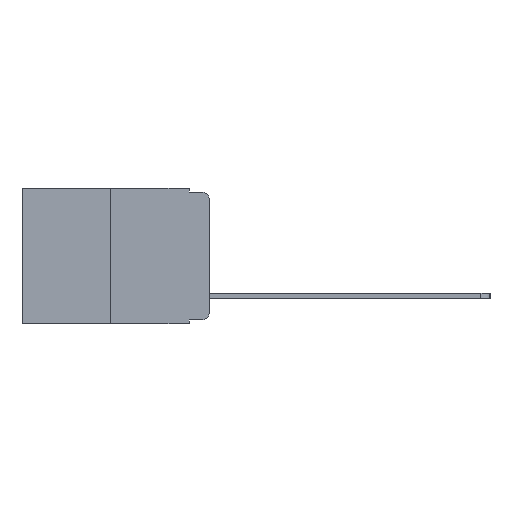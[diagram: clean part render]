
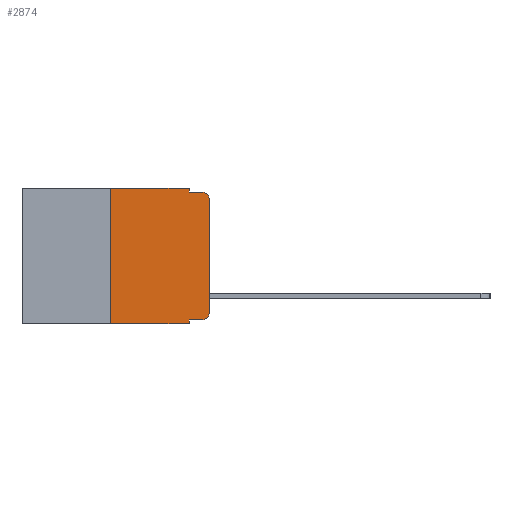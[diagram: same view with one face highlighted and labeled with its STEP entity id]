
A CAD part, left-side view. The second image highlights one B-rep face of the part: STEP entity #2874.
In plain terms, the highlighted planar face has unit normal (-1, 0, 0).
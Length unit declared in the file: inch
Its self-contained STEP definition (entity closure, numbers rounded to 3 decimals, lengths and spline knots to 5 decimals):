
#144 = VERTEX_POINT ( 'NONE', #8713 ) ;
#613 = AXIS2_PLACEMENT_3D ( 'NONE', #4782, #10572, #5807 ) ;
#1091 = DIRECTION ( 'NONE',  ( 0., 0., 1. ) ) ;
#1353 = VERTEX_POINT ( 'NONE', #3921 ) ;
#1379 = AXIS2_PLACEMENT_3D ( 'NONE', #8237, #2510, #9073 ) ;
#1394 = EDGE_CURVE ( 'NONE', #1538, #8094, #6703, .T. ) ;
#1402 = DIRECTION ( 'NONE',  ( 0., 0., -1. ) ) ;
#1431 = VECTOR ( 'NONE', #1402, 39.37008 ) ;
#1538 = VERTEX_POINT ( 'NONE', #11874 ) ;
#1625 = LINE ( 'NONE', #11151, #7016 ) ;
#1773 = CARTESIAN_POINT ( 'NONE',  ( 0., 0.25, 0. ) ) ;
#1789 = VECTOR ( 'NONE', #8537, 39.37008 ) ;
#2220 = CARTESIAN_POINT ( 'NONE',  ( 0., 0.051, -0.343 ) ) ;
#2510 = DIRECTION ( 'NONE',  ( -1., 0., 0. ) ) ;
#2740 = ORIENTED_EDGE ( 'NONE', *, *, #9240, .T. ) ;
#2832 = VERTEX_POINT ( 'NONE', #3524 ) ;
#2874 = ADVANCED_FACE ( 'NONE', ( #10399 ), #11400, .F. ) ;
#3105 = VERTEX_POINT ( 'NONE', #7857 ) ;
#3524 = CARTESIAN_POINT ( 'NONE',  ( 0., 0.051, -0.01 ) ) ;
#3537 = CARTESIAN_POINT ( 'NONE',  ( 0., 0.473, 0. ) ) ;
#3663 = DIRECTION ( 'NONE',  ( 0., -1., 0. ) ) ;
#3921 = CARTESIAN_POINT ( 'NONE',  ( 0., 0.25, -0.343 ) ) ;
#4570 = VERTEX_POINT ( 'NONE', #2220 ) ;
#4718 = VERTEX_POINT ( 'NONE', #5042 ) ;
#4782 = CARTESIAN_POINT ( 'NONE',  ( 0., 0.02, -0.313 ) ) ;
#4813 = CIRCLE ( 'NONE', #1379, 0.02 ) ;
#4841 = LINE ( 'NONE', #1773, #1789 ) ;
#4926 = VERTEX_POINT ( 'NONE', #9681 ) ;
#5042 = CARTESIAN_POINT ( 'NONE',  ( 0., 0.02, -0.333 ) ) ;
#5122 = DIRECTION ( 'NONE',  ( 0., 0., -1. ) ) ;
#5158 = LINE ( 'NONE', #6201, #9299 ) ;
#5350 = LINE ( 'NONE', #7892, #9925 ) ;
#5552 = DIRECTION ( 'NONE',  ( 0., -1., 0. ) ) ;
#5628 = VECTOR ( 'NONE', #9993, 39.37008 ) ;
#5807 = DIRECTION ( 'NONE',  ( 0., 0., -1. ) ) ;
#6201 = CARTESIAN_POINT ( 'NONE',  ( 0., 0.051, -0.333 ) ) ;
#6703 = LINE ( 'NONE', #3537, #8365 ) ;
#6775 = CARTESIAN_POINT ( 'NONE',  ( 0., 0.051, 0. ) ) ;
#6831 = EDGE_CURVE ( 'NONE', #1353, #4570, #5350, .T. ) ;
#6885 = LINE ( 'NONE', #7373, #1431 ) ;
#6988 = DIRECTION ( 'NONE',  ( 0., -1., 0. ) ) ;
#7016 = VECTOR ( 'NONE', #5552, 39.37008 ) ;
#7077 = ORIENTED_EDGE ( 'NONE', *, *, #10727, .F. ) ;
#7215 = ORIENTED_EDGE ( 'NONE', *, *, #1394, .F. ) ;
#7242 = ORIENTED_EDGE ( 'NONE', *, *, #11095, .F. ) ;
#7373 = CARTESIAN_POINT ( 'NONE',  ( 0., 0.051, 0. ) ) ;
#7407 = ORIENTED_EDGE ( 'NONE', *, *, #10118, .T. ) ;
#7424 = ORIENTED_EDGE ( 'NONE', *, *, #6831, .T. ) ;
#7665 = ORIENTED_EDGE ( 'NONE', *, *, #10475, .F. ) ;
#7838 = VERTEX_POINT ( 'NONE', #9892 ) ;
#7857 = CARTESIAN_POINT ( 'NONE',  ( 0., 0., -0.313 ) ) ;
#7892 = CARTESIAN_POINT ( 'NONE',  ( 0., 0.473, -0.343 ) ) ;
#8013 = ORIENTED_EDGE ( 'NONE', *, *, #10121, .F. ) ;
#8094 = VERTEX_POINT ( 'NONE', #8423 ) ;
#8237 = CARTESIAN_POINT ( 'NONE',  ( 0., 0.02, -0.03 ) ) ;
#8365 = VECTOR ( 'NONE', #3663, 39.37008 ) ;
#8423 = CARTESIAN_POINT ( 'NONE',  ( 0., 0.051, 0. ) ) ;
#8537 = DIRECTION ( 'NONE',  ( 0., 0., 1. ) ) ;
#8713 = CARTESIAN_POINT ( 'NONE',  ( 0., 0., -0.03 ) ) ;
#8810 = ORIENTED_EDGE ( 'NONE', *, *, #10085, .T. ) ;
#8917 = ORIENTED_EDGE ( 'NONE', *, *, #10070, .T. ) ;
#9073 = DIRECTION ( 'NONE',  ( 0., 0., -1. ) ) ;
#9098 = AXIS2_PLACEMENT_3D ( 'NONE', #11641, #11711, #5122 ) ;
#9240 = EDGE_CURVE ( 'NONE', #3105, #144, #10032, .T. ) ;
#9299 = VECTOR ( 'NONE', #6988, 39.37008 ) ;
#9528 = DIRECTION ( 'NONE',  ( 0., -1., 0. ) ) ;
#9681 = CARTESIAN_POINT ( 'NONE',  ( 0., 0.02, -0.01 ) ) ;
#9892 = CARTESIAN_POINT ( 'NONE',  ( 0., 0.051, -0.333 ) ) ;
#9925 = VECTOR ( 'NONE', #9528, 39.37008 ) ;
#9993 = DIRECTION ( 'NONE',  ( 0., 0., -1. ) ) ;
#10032 = LINE ( 'NONE', #11964, #11894 ) ;
#10070 = EDGE_CURVE ( 'NONE', #7838, #4718, #5158, .T. ) ;
#10085 = EDGE_CURVE ( 'NONE', #4718, #3105, #11381, .T. ) ;
#10118 = EDGE_CURVE ( 'NONE', #144, #4926, #4813, .T. ) ;
#10121 = EDGE_CURVE ( 'NONE', #7838, #4570, #6885, .T. ) ;
#10145 = LINE ( 'NONE', #6775, #5628 ) ;
#10399 = FACE_OUTER_BOUND ( 'NONE', #10762, .T. ) ;
#10475 = EDGE_CURVE ( 'NONE', #8094, #2832, #10145, .T. ) ;
#10572 = DIRECTION ( 'NONE',  ( -1., 0., 0. ) ) ;
#10727 = EDGE_CURVE ( 'NONE', #1353, #1538, #4841, .T. ) ;
#10762 = EDGE_LOOP ( 'NONE', ( #2740, #7407, #7242, #7665, #7215, #7077, #7424, #8013, #8917, #8810 ) ) ;
#11095 = EDGE_CURVE ( 'NONE', #2832, #4926, #1625, .T. ) ;
#11151 = CARTESIAN_POINT ( 'NONE',  ( 0., 0.051, -0.01 ) ) ;
#11381 = CIRCLE ( 'NONE', #613, 0.02 ) ;
#11400 = PLANE ( 'NONE',  #9098 ) ;
#11641 = CARTESIAN_POINT ( 'NONE',  ( 0., 0.473, 0. ) ) ;
#11711 = DIRECTION ( 'NONE',  ( 1., 0., 0. ) ) ;
#11874 = CARTESIAN_POINT ( 'NONE',  ( 0., 0.25, 0. ) ) ;
#11894 = VECTOR ( 'NONE', #1091, 39.37008 ) ;
#11964 = CARTESIAN_POINT ( 'NONE',  ( 0., 0., 0. ) ) ;
